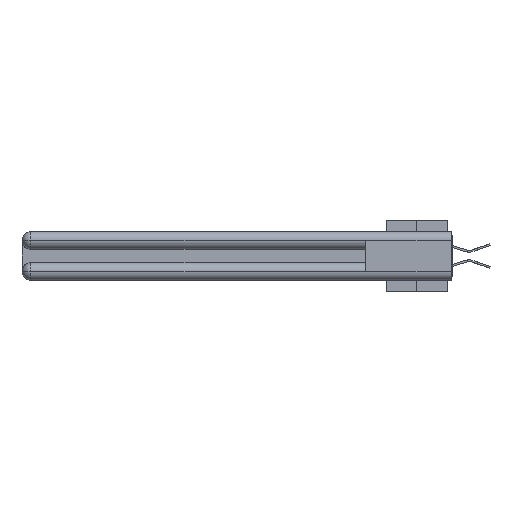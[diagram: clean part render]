
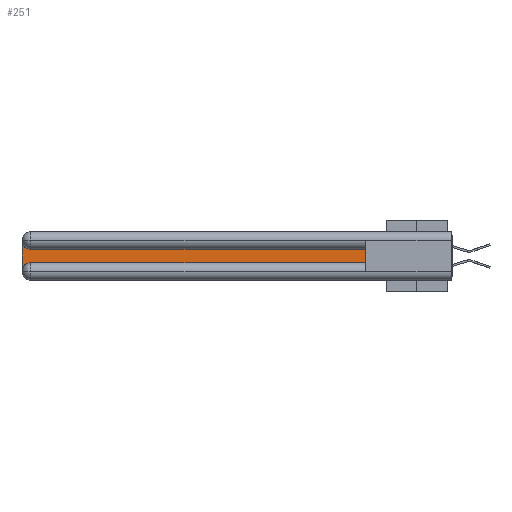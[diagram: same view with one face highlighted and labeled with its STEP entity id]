
A CAD part, left-side view. The second image highlights one B-rep face of the part: STEP entity #251.
In plain terms, the highlighted planar face has unit normal (-1, 0, 0).
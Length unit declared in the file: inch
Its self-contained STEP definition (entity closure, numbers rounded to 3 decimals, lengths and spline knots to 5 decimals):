
#251 = ADVANCED_FACE ( 'NONE', ( #25272 ), #19389, .F. ) ;
#499 = DIRECTION ( 'NONE',  ( 1., 0., 0. ) ) ;
#890 = CARTESIAN_POINT ( 'NONE',  ( 0.075, 2.94, -0.0625 ) ) ;
#1058 = CARTESIAN_POINT ( 'NONE',  ( 0.075, 0.6, -0.1225 ) ) ;
#1739 = AXIS2_PLACEMENT_3D ( 'NONE', #33865, #28162, #34221 ) ;
#1903 = VERTEX_POINT ( 'NONE', #12503 ) ;
#1967 = CARTESIAN_POINT ( 'NONE',  ( 0.075, 3., -0.0625 ) ) ;
#4391 = CARTESIAN_POINT ( 'NONE',  ( 0.075, 2.94, -0.2775 ) ) ;
#4854 = ORIENTED_EDGE ( 'NONE', *, *, #28628, .T. ) ;
#5543 = DIRECTION ( 'NONE',  ( 0., -1., 0. ) ) ;
#5591 = CARTESIAN_POINT ( 'NONE',  ( 0.075, 0.6, -0.2175 ) ) ;
#6677 = VERTEX_POINT ( 'NONE', #14894 ) ;
#7099 = DIRECTION ( 'NONE',  ( 0., 0., -1. ) ) ;
#9263 = VECTOR ( 'NONE', #16337, 39.37008 ) ;
#9612 = DIRECTION ( 'NONE',  ( 0., 0., -1. ) ) ;
#10571 = CARTESIAN_POINT ( 'NONE',  ( 0.075, 0.6, -0.2175 ) ) ;
#11673 = EDGE_CURVE ( 'NONE', #35292, #35409, #25827, .T. ) ;
#12022 = CARTESIAN_POINT ( 'NONE',  ( 0.075, 3., -0.2175 ) ) ;
#12503 = CARTESIAN_POINT ( 'NONE',  ( 0.075, 3., -0.2775 ) ) ;
#14383 = ORIENTED_EDGE ( 'NONE', *, *, #34392, .T. ) ;
#14894 = CARTESIAN_POINT ( 'NONE',  ( 0.075, 2.94, -0.1225 ) ) ;
#15052 = LINE ( 'NONE', #12022, #29822 ) ;
#15946 = AXIS2_PLACEMENT_3D ( 'NONE', #890, #499, #9612 ) ;
#16337 = DIRECTION ( 'NONE',  ( 0., 0., 1. ) ) ;
#17306 = VERTEX_POINT ( 'NONE', #26768 ) ;
#18024 = ORIENTED_EDGE ( 'NONE', *, *, #30541, .T. ) ;
#18888 = CIRCLE ( 'NONE', #15946, 0.06 ) ;
#19389 = PLANE ( 'NONE',  #1739 ) ;
#21851 = DIRECTION ( 'NONE',  ( 1., 0., 0. ) ) ;
#22429 = ORIENTED_EDGE ( 'NONE', *, *, #28701, .T. ) ;
#22677 = EDGE_CURVE ( 'NONE', #37446, #1903, #15052, .T. ) ;
#23039 = CARTESIAN_POINT ( 'NONE',  ( 0.075, 0.6, -0.1225 ) ) ;
#23043 = LINE ( 'NONE', #5591, #29559 ) ;
#24309 = EDGE_LOOP ( 'NONE', ( #4854, #14383, #32358, #18024, #22429, #32001 ) ) ;
#25272 = FACE_OUTER_BOUND ( 'NONE', #24309, .T. ) ;
#25827 = LINE ( 'NONE', #10571, #9263 ) ;
#26768 = CARTESIAN_POINT ( 'NONE',  ( 0.075, 2.94, -0.2175 ) ) ;
#28162 = DIRECTION ( 'NONE',  ( 1., 0., 0. ) ) ;
#28628 = EDGE_CURVE ( 'NONE', #35409, #6677, #32801, .T. ) ;
#28701 = EDGE_CURVE ( 'NONE', #17306, #35292, #23043, .T. ) ;
#29413 = CIRCLE ( 'NONE', #31909, 0.06 ) ;
#29559 = VECTOR ( 'NONE', #5543, 39.37008 ) ;
#29822 = VECTOR ( 'NONE', #35993, 39.37008 ) ;
#30541 = EDGE_CURVE ( 'NONE', #1903, #17306, #29413, .T. ) ;
#31909 = AXIS2_PLACEMENT_3D ( 'NONE', #4391, #21851, #7099 ) ;
#32001 = ORIENTED_EDGE ( 'NONE', *, *, #11673, .T. ) ;
#32337 = DIRECTION ( 'NONE',  ( 0., 1., 0. ) ) ;
#32358 = ORIENTED_EDGE ( 'NONE', *, *, #22677, .T. ) ;
#32801 = LINE ( 'NONE', #23039, #36942 ) ;
#33865 = CARTESIAN_POINT ( 'NONE',  ( 0.075, 3., -0.1225 ) ) ;
#34221 = DIRECTION ( 'NONE',  ( 0., 0., -1. ) ) ;
#34392 = EDGE_CURVE ( 'NONE', #6677, #37446, #18888, .T. ) ;
#35292 = VERTEX_POINT ( 'NONE', #38177 ) ;
#35409 = VERTEX_POINT ( 'NONE', #1058 ) ;
#35993 = DIRECTION ( 'NONE',  ( 0., 0., -1. ) ) ;
#36942 = VECTOR ( 'NONE', #32337, 39.37008 ) ;
#37446 = VERTEX_POINT ( 'NONE', #1967 ) ;
#38177 = CARTESIAN_POINT ( 'NONE',  ( 0.075, 0.6, -0.2175 ) ) ;
